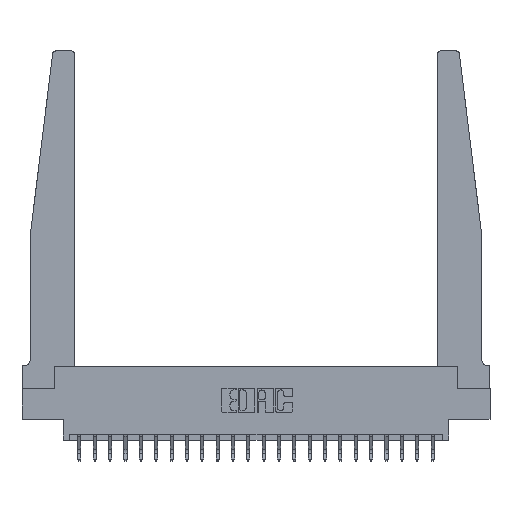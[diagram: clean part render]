
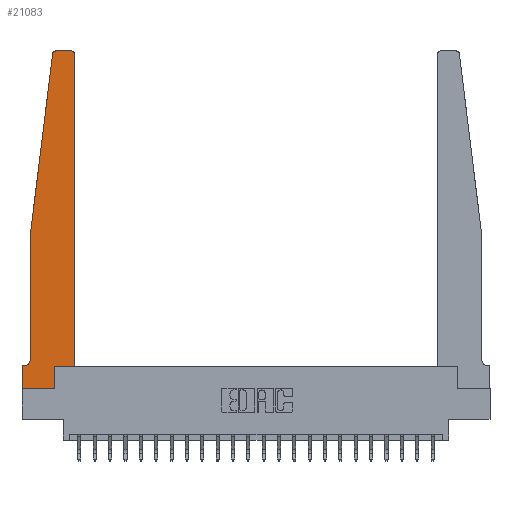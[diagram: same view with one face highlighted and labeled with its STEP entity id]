
A CAD part, top view. The second image highlights one B-rep face of the part: STEP entity #21083.
In plain terms, the highlighted planar face has unit normal (0, 0, 1).
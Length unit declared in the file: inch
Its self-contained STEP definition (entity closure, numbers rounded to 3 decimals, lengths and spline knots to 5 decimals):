
#28 = CIRCLE ( 'NONE', #18990, 0.03 ) ;
#177 = CARTESIAN_POINT ( 'NONE',  ( 0.2605, 0.18, 0.37 ) ) ;
#257 = AXIS2_PLACEMENT_3D ( 'NONE', #22903, #13986, #3251 ) ;
#268 = CARTESIAN_POINT ( 'NONE',  ( 0.425, 0.18, 0.37 ) ) ;
#883 = CARTESIAN_POINT ( 'NONE',  ( 0., 0.1875, 0.37 ) ) ;
#964 = ORIENTED_EDGE ( 'NONE', *, *, #2016, .T. ) ;
#1049 = ORIENTED_EDGE ( 'NONE', *, *, #22787, .T. ) ;
#1094 = DIRECTION ( 'NONE',  ( 1., 0., 0. ) ) ;
#1321 = DIRECTION ( 'NONE',  ( -1., 0., 0. ) ) ;
#1411 = PLANE ( 'NONE',  #257 ) ;
#1707 = EDGE_CURVE ( 'NONE', #2948, #20683, #12534, .T. ) ;
#2003 = DIRECTION ( 'NONE',  ( 0., 1., 0. ) ) ;
#2016 = EDGE_CURVE ( 'NONE', #17100, #16941, #7496, .T. ) ;
#2948 = VERTEX_POINT ( 'NONE', #9615 ) ;
#2956 = ORIENTED_EDGE ( 'NONE', *, *, #1707, .T. ) ;
#3072 = CARTESIAN_POINT ( 'NONE',  ( 0.25, 2.75, 0.37 ) ) ;
#3102 = EDGE_CURVE ( 'NONE', #12903, #6159, #14150, .T. ) ;
#3251 = DIRECTION ( 'NONE',  ( 1., 0., 0. ) ) ;
#3549 = CARTESIAN_POINT ( 'NONE',  ( 0., 0., 0.37 ) ) ;
#3701 = ORIENTED_EDGE ( 'NONE', *, *, #17818, .T. ) ;
#3744 = ORIENTED_EDGE ( 'NONE', *, *, #8812, .T. ) ;
#3761 = DIRECTION ( 'NONE',  ( 0., 0., -1. ) ) ;
#3765 = DIRECTION ( 'NONE',  ( 1., 0., 0. ) ) ;
#4385 = CARTESIAN_POINT ( 'NONE',  ( 0.27653, 2.72, 0.37 ) ) ;
#4940 = VECTOR ( 'NONE', #20022, 39.37008 ) ;
#4949 = VERTEX_POINT ( 'NONE', #15510 ) ;
#4974 = VECTOR ( 'NONE', #11979, 39.37008 ) ;
#5509 = LINE ( 'NONE', #5948, #9736 ) ;
#5948 = CARTESIAN_POINT ( 'NONE',  ( 0., 0., 0.37 ) ) ;
#6138 = VERTEX_POINT ( 'NONE', #22723 ) ;
#6159 = VERTEX_POINT ( 'NONE', #17435 ) ;
#6196 = DIRECTION ( 'NONE',  ( 1., 0., 0. ) ) ;
#6867 = VERTEX_POINT ( 'NONE', #12923 ) ;
#7393 = ORIENTED_EDGE ( 'NONE', *, *, #11972, .T. ) ;
#7478 = VECTOR ( 'NONE', #1321, 39.37008 ) ;
#7496 = LINE ( 'NONE', #19849, #21216 ) ;
#8049 = LINE ( 'NONE', #3072, #7478 ) ;
#8441 = ORIENTED_EDGE ( 'NONE', *, *, #15210, .T. ) ;
#8511 = EDGE_CURVE ( 'NONE', #6159, #17100, #20379, .T. ) ;
#8812 = EDGE_CURVE ( 'NONE', #11742, #13444, #9759, .T. ) ;
#9296 = EDGE_CURVE ( 'NONE', #20683, #12903, #5509, .T. ) ;
#9441 = EDGE_CURVE ( 'NONE', #6138, #21838, #8049, .T. ) ;
#9550 = DIRECTION ( 'NONE',  ( 0., 0., 1. ) ) ;
#9615 = CARTESIAN_POINT ( 'NONE',  ( 0.015, 0.1875, 0.37 ) ) ;
#9736 = VECTOR ( 'NONE', #20291, 39.37008 ) ;
#9759 = LINE ( 'NONE', #10184, #4974 ) ;
#9999 = FACE_OUTER_BOUND ( 'NONE', #10012, .T. ) ;
#10012 = EDGE_LOOP ( 'NONE', ( #22036, #3701, #3744, #11185, #7393, #2956, #10187, #20131, #16827, #964, #8441, #1049 ) ) ;
#10184 = CARTESIAN_POINT ( 'NONE',  ( 0.065, 1.25, 0.37 ) ) ;
#10187 = ORIENTED_EDGE ( 'NONE', *, *, #9296, .T. ) ;
#10783 = AXIS2_PLACEMENT_3D ( 'NONE', #4385, #16923, #6196 ) ;
#11185 = ORIENTED_EDGE ( 'NONE', *, *, #21647, .T. ) ;
#11251 = CIRCLE ( 'NONE', #14010, 0.05 ) ;
#11417 = VECTOR ( 'NONE', #20930, 39.37008 ) ;
#11742 = VERTEX_POINT ( 'NONE', #19005 ) ;
#11972 = EDGE_CURVE ( 'NONE', #4949, #2948, #11251, .T. ) ;
#11979 = DIRECTION ( 'NONE',  ( -0.122, -0.992, 0. ) ) ;
#11998 = CARTESIAN_POINT ( 'NONE',  ( 0.065, 0.1875, 0.37 ) ) ;
#12534 = LINE ( 'NONE', #11998, #11417 ) ;
#12903 = VERTEX_POINT ( 'NONE', #3549 ) ;
#12923 = CARTESIAN_POINT ( 'NONE',  ( 0.425, 2.72, 0.37 ) ) ;
#13103 = CARTESIAN_POINT ( 'NONE',  ( 0.2605, 0.18, 0.37 ) ) ;
#13444 = VERTEX_POINT ( 'NONE', #21008 ) ;
#13669 = CARTESIAN_POINT ( 'NONE',  ( 0., 0., 0.37 ) ) ;
#13986 = DIRECTION ( 'NONE',  ( 0., 0., 1. ) ) ;
#14010 = AXIS2_PLACEMENT_3D ( 'NONE', #14490, #3761, #16293 ) ;
#14150 = LINE ( 'NONE', #13669, #18393 ) ;
#14190 = CARTESIAN_POINT ( 'NONE',  ( 0.27653, 2.75, 0.37 ) ) ;
#14362 = CARTESIAN_POINT ( 'NONE',  ( 0.425, 0.18, 0.37 ) ) ;
#14468 = LINE ( 'NONE', #268, #4940 ) ;
#14490 = CARTESIAN_POINT ( 'NONE',  ( 0.015, 0.2375, 0.37 ) ) ;
#15210 = EDGE_CURVE ( 'NONE', #16941, #6867, #14468, .T. ) ;
#15510 = CARTESIAN_POINT ( 'NONE',  ( 0.065, 0.2375, 0.37 ) ) ;
#15606 = VECTOR ( 'NONE', #2003, 39.37008 ) ;
#16293 = DIRECTION ( 'NONE',  ( -1., 0., 0. ) ) ;
#16827 = ORIENTED_EDGE ( 'NONE', *, *, #8511, .T. ) ;
#16923 = DIRECTION ( 'NONE',  ( 0., 0., 1. ) ) ;
#16941 = VERTEX_POINT ( 'NONE', #14362 ) ;
#17100 = VERTEX_POINT ( 'NONE', #13103 ) ;
#17435 = CARTESIAN_POINT ( 'NONE',  ( 0.2605, 0., 0.37 ) ) ;
#17818 = EDGE_CURVE ( 'NONE', #21838, #11742, #19739, .T. ) ;
#18393 = VECTOR ( 'NONE', #1094, 39.37008 ) ;
#18401 = LINE ( 'NONE', #19104, #22549 ) ;
#18990 = AXIS2_PLACEMENT_3D ( 'NONE', #20296, #9550, #22055 ) ;
#19005 = CARTESIAN_POINT ( 'NONE',  ( 0.24675, 2.72367, 0.37 ) ) ;
#19104 = CARTESIAN_POINT ( 'NONE',  ( 0.065, 1.25, 0.37 ) ) ;
#19739 = CIRCLE ( 'NONE', #10783, 0.03 ) ;
#19849 = CARTESIAN_POINT ( 'NONE',  ( 0.425, 0.18, 0.37 ) ) ;
#20022 = DIRECTION ( 'NONE',  ( 0., 1., 0. ) ) ;
#20131 = ORIENTED_EDGE ( 'NONE', *, *, #3102, .T. ) ;
#20291 = DIRECTION ( 'NONE',  ( 0., -1., 0. ) ) ;
#20296 = CARTESIAN_POINT ( 'NONE',  ( 0.395, 2.72, 0.37 ) ) ;
#20379 = LINE ( 'NONE', #177, #15606 ) ;
#20683 = VERTEX_POINT ( 'NONE', #883 ) ;
#20930 = DIRECTION ( 'NONE',  ( -1., 0., 0. ) ) ;
#21008 = CARTESIAN_POINT ( 'NONE',  ( 0.065, 1.25, 0.37 ) ) ;
#21083 = ADVANCED_FACE ( 'NONE', ( #9999 ), #1411, .T. ) ;
#21216 = VECTOR ( 'NONE', #3765, 39.37008 ) ;
#21647 = EDGE_CURVE ( 'NONE', #13444, #4949, #18401, .T. ) ;
#21838 = VERTEX_POINT ( 'NONE', #14190 ) ;
#22036 = ORIENTED_EDGE ( 'NONE', *, *, #9441, .T. ) ;
#22055 = DIRECTION ( 'NONE',  ( 1., 0., 0. ) ) ;
#22549 = VECTOR ( 'NONE', #22648, 39.37008 ) ;
#22648 = DIRECTION ( 'NONE',  ( 0., -1., 0. ) ) ;
#22723 = CARTESIAN_POINT ( 'NONE',  ( 0.395, 2.75, 0.37 ) ) ;
#22787 = EDGE_CURVE ( 'NONE', #6867, #6138, #28, .T. ) ;
#22903 = CARTESIAN_POINT ( 'NONE',  ( 0., 0.1875, 0.37 ) ) ;
